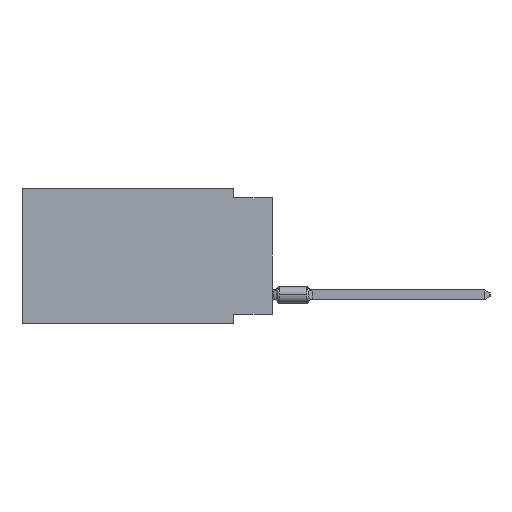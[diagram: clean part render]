
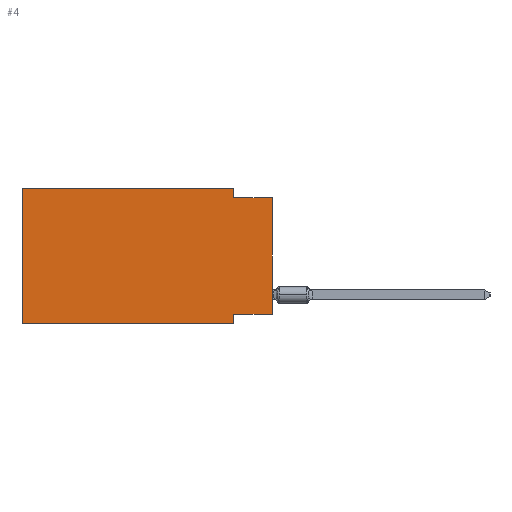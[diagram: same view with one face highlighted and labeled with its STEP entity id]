
A CAD part, left-side view. The second image highlights one B-rep face of the part: STEP entity #4.
In plain terms, the highlighted planar face has unit normal (-1, 0, 0).
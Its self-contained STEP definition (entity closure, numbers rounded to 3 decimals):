
#4 = ADVANCED_FACE ( 'NONE', ( #28466 ), #51934, .F. ) ;
#491 = DIRECTION ( 'NONE',  ( 0., 0., 1. ) ) ;
#493 = LINE ( 'NONE', #28184, #34676 ) ;
#1960 = EDGE_CURVE ( 'NONE', #40715, #29680, #31515, .T. ) ;
#2767 = EDGE_CURVE ( 'NONE', #12112, #23644, #46939, .T. ) ;
#2978 = EDGE_CURVE ( 'NONE', #41266, #18157, #34422, .T. ) ;
#3335 = VECTOR ( 'NONE', #35274, 1000. ) ;
#4070 = ORIENTED_EDGE ( 'NONE', *, *, #1960, .F. ) ;
#4495 = DIRECTION ( 'NONE',  ( 1., 0., 0. ) ) ;
#6962 = VECTOR ( 'NONE', #28071, 1000. ) ;
#7270 = ORIENTED_EDGE ( 'NONE', *, *, #16099, .F. ) ;
#7864 = LINE ( 'NONE', #15234, #19177 ) ;
#8309 = CARTESIAN_POINT ( 'NONE',  ( 0., 2.54, 0. ) ) ;
#10036 = CARTESIAN_POINT ( 'NONE',  ( 0., 16.383, -8.89 ) ) ;
#11487 = DIRECTION ( 'NONE',  ( 0., -1., 0. ) ) ;
#11621 = DIRECTION ( 'NONE',  ( 0., 0., -1. ) ) ;
#11832 = EDGE_CURVE ( 'NONE', #15412, #25259, #7864, .T. ) ;
#12112 = VERTEX_POINT ( 'NONE', #42080 ) ;
#12939 = CARTESIAN_POINT ( 'NONE',  ( 0., 2.54, -8.255 ) ) ;
#13274 = EDGE_CURVE ( 'NONE', #25259, #18157, #493, .T. ) ;
#13319 = VECTOR ( 'NONE', #37866, 1000. ) ;
#15234 = CARTESIAN_POINT ( 'NONE',  ( 0., 0., -8.255 ) ) ;
#15412 = VERTEX_POINT ( 'NONE', #17281 ) ;
#16099 = EDGE_CURVE ( 'NONE', #41266, #12112, #33187, .T. ) ;
#16498 = CARTESIAN_POINT ( 'NONE',  ( 0., 2.54, -0.635 ) ) ;
#16829 = VECTOR ( 'NONE', #491, 1000. ) ;
#17245 = ORIENTED_EDGE ( 'NONE', *, *, #2767, .F. ) ;
#17281 = CARTESIAN_POINT ( 'NONE',  ( 0., 0., -8.255 ) ) ;
#17484 = VECTOR ( 'NONE', #26631, 1000. ) ;
#18157 = VERTEX_POINT ( 'NONE', #29010 ) ;
#18606 = ORIENTED_EDGE ( 'NONE', *, *, #13274, .F. ) ;
#19177 = VECTOR ( 'NONE', #19710, 1000. ) ;
#19710 = DIRECTION ( 'NONE',  ( 0., 1., 0. ) ) ;
#21579 = AXIS2_PLACEMENT_3D ( 'NONE', #44567, #4495, #11621 ) ;
#23107 = CARTESIAN_POINT ( 'NONE',  ( 0., 2.54, 0. ) ) ;
#23644 = VERTEX_POINT ( 'NONE', #23107 ) ;
#24187 = CARTESIAN_POINT ( 'NONE',  ( 0., 0., 0. ) ) ;
#25259 = VERTEX_POINT ( 'NONE', #12939 ) ;
#25603 = ORIENTED_EDGE ( 'NONE', *, *, #11832, .F. ) ;
#25736 = EDGE_LOOP ( 'NONE', ( #46781, #4070, #35331, #17245, #7270, #41838, #18606, #25603 ) ) ;
#26612 = EDGE_CURVE ( 'NONE', #23644, #40715, #32034, .T. ) ;
#26631 = DIRECTION ( 'NONE',  ( 0., -1., 0. ) ) ;
#28071 = DIRECTION ( 'NONE',  ( 0., 0., -1. ) ) ;
#28184 = CARTESIAN_POINT ( 'NONE',  ( 0., 2.54, -8.89 ) ) ;
#28466 = FACE_OUTER_BOUND ( 'NONE', #25736, .T. ) ;
#29010 = CARTESIAN_POINT ( 'NONE',  ( 0., 2.54, -8.89 ) ) ;
#29680 = VERTEX_POINT ( 'NONE', #44241 ) ;
#29682 = EDGE_CURVE ( 'NONE', #15412, #29680, #43720, .T. ) ;
#31515 = LINE ( 'NONE', #47594, #42845 ) ;
#31888 = DIRECTION ( 'NONE',  ( 0., 0., -1. ) ) ;
#32034 = LINE ( 'NONE', #8309, #6962 ) ;
#33187 = LINE ( 'NONE', #48487, #16829 ) ;
#34422 = LINE ( 'NONE', #34940, #13319 ) ;
#34676 = VECTOR ( 'NONE', #31888, 1000. ) ;
#34940 = CARTESIAN_POINT ( 'NONE',  ( 0., 16.383, -8.89 ) ) ;
#35274 = DIRECTION ( 'NONE',  ( 0., 0., 1. ) ) ;
#35331 = ORIENTED_EDGE ( 'NONE', *, *, #26612, .F. ) ;
#37866 = DIRECTION ( 'NONE',  ( 0., -1., 0. ) ) ;
#38507 = CARTESIAN_POINT ( 'NONE',  ( 0., 16.383, 0. ) ) ;
#40715 = VERTEX_POINT ( 'NONE', #16498 ) ;
#41266 = VERTEX_POINT ( 'NONE', #10036 ) ;
#41838 = ORIENTED_EDGE ( 'NONE', *, *, #2978, .T. ) ;
#42080 = CARTESIAN_POINT ( 'NONE',  ( 0., 16.383, 0. ) ) ;
#42845 = VECTOR ( 'NONE', #11487, 1000. ) ;
#43720 = LINE ( 'NONE', #24187, #3335 ) ;
#44241 = CARTESIAN_POINT ( 'NONE',  ( 0., 0., -0.635 ) ) ;
#44567 = CARTESIAN_POINT ( 'NONE',  ( 0., 16.383, 0. ) ) ;
#46781 = ORIENTED_EDGE ( 'NONE', *, *, #29682, .T. ) ;
#46939 = LINE ( 'NONE', #38507, #17484 ) ;
#47594 = CARTESIAN_POINT ( 'NONE',  ( 0., 0., -0.635 ) ) ;
#48487 = CARTESIAN_POINT ( 'NONE',  ( 0., 16.383, 0. ) ) ;
#51934 = PLANE ( 'NONE',  #21579 ) ;
